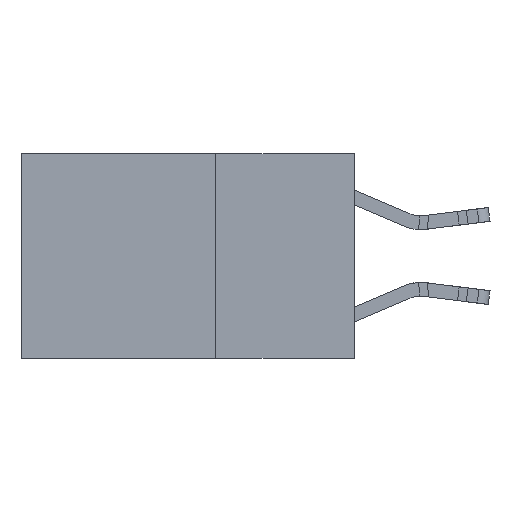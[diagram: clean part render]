
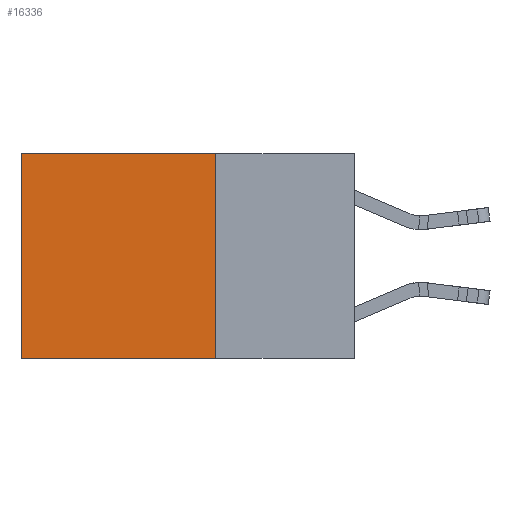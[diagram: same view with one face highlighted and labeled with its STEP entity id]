
A CAD part, left-side view. The second image highlights one B-rep face of the part: STEP entity #16336.
In plain terms, the highlighted planar face has unit normal (-1, 0, 0).
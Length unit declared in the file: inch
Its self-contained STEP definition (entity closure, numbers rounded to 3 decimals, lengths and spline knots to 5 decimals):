
#178 = VECTOR ( 'NONE', #10532, 39.37008 ) ;
#2789 = CARTESIAN_POINT ( 'NONE',  ( 0.2625, 0.25, 0. ) ) ;
#3501 = LINE ( 'NONE', #3801, #26653 ) ;
#3801 = CARTESIAN_POINT ( 'NONE',  ( 0.2625, 0.25, 0. ) ) ;
#4368 = CARTESIAN_POINT ( 'NONE',  ( 0.2625, 0.6, 0. ) ) ;
#4740 = CARTESIAN_POINT ( 'NONE',  ( 0.2625, 0.25, -0.37 ) ) ;
#4819 = CARTESIAN_POINT ( 'NONE',  ( 0.2625, 0.6, -0.37 ) ) ;
#5310 = ORIENTED_EDGE ( 'NONE', *, *, #27569, .F. ) ;
#6017 = DIRECTION ( 'NONE',  ( 0., 0., -1. ) ) ;
#7129 = ORIENTED_EDGE ( 'NONE', *, *, #21452, .F. ) ;
#7217 = DIRECTION ( 'NONE',  ( 0., 0., -1. ) ) ;
#8449 = LINE ( 'NONE', #10957, #178 ) ;
#8516 = LINE ( 'NONE', #4368, #26164 ) ;
#9610 = LINE ( 'NONE', #4740, #10892 ) ;
#10532 = DIRECTION ( 'NONE',  ( 0., 1., 0. ) ) ;
#10892 = VECTOR ( 'NONE', #20687, 39.37008 ) ;
#10957 = CARTESIAN_POINT ( 'NONE',  ( 0.2625, 0.25, 0. ) ) ;
#11233 = EDGE_LOOP ( 'NONE', ( #13045, #7129, #5310, #15341 ) ) ;
#11630 = VERTEX_POINT ( 'NONE', #19856 ) ;
#12531 = CARTESIAN_POINT ( 'NONE',  ( 0.2625, 0.6, 0. ) ) ;
#13045 = ORIENTED_EDGE ( 'NONE', *, *, #26352, .T. ) ;
#14764 = CARTESIAN_POINT ( 'NONE',  ( 0.2625, 0.25, 0. ) ) ;
#15341 = ORIENTED_EDGE ( 'NONE', *, *, #27262, .T. ) ;
#16336 = ADVANCED_FACE ( 'NONE', ( #16425 ), #18478, .F. ) ;
#16425 = FACE_OUTER_BOUND ( 'NONE', #11233, .T. ) ;
#18478 = PLANE ( 'NONE',  #19723 ) ;
#19723 = AXIS2_PLACEMENT_3D ( 'NONE', #2789, #27493, #7217 ) ;
#19856 = CARTESIAN_POINT ( 'NONE',  ( 0.2625, 0.25, -0.37 ) ) ;
#20687 = DIRECTION ( 'NONE',  ( 0., 1., 0. ) ) ;
#21381 = DIRECTION ( 'NONE',  ( 0., 0., -1. ) ) ;
#21452 = EDGE_CURVE ( 'NONE', #11630, #28590, #9610, .T. ) ;
#21998 = VERTEX_POINT ( 'NONE', #14764 ) ;
#26164 = VECTOR ( 'NONE', #6017, 39.37008 ) ;
#26244 = VERTEX_POINT ( 'NONE', #12531 ) ;
#26352 = EDGE_CURVE ( 'NONE', #26244, #28590, #8516, .T. ) ;
#26653 = VECTOR ( 'NONE', #21381, 39.37008 ) ;
#27262 = EDGE_CURVE ( 'NONE', #21998, #26244, #8449, .T. ) ;
#27493 = DIRECTION ( 'NONE',  ( 1., 0., 0. ) ) ;
#27569 = EDGE_CURVE ( 'NONE', #21998, #11630, #3501, .T. ) ;
#28590 = VERTEX_POINT ( 'NONE', #4819 ) ;
